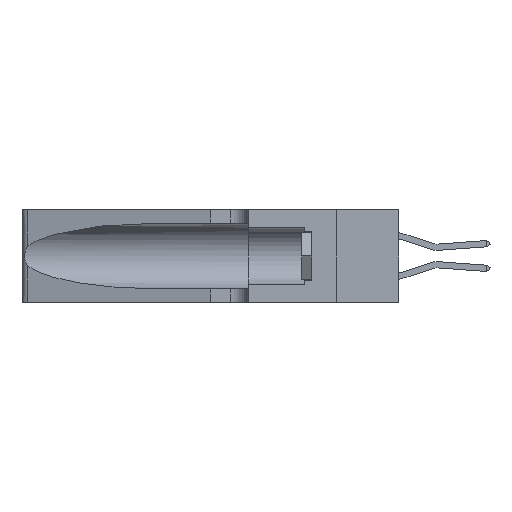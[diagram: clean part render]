
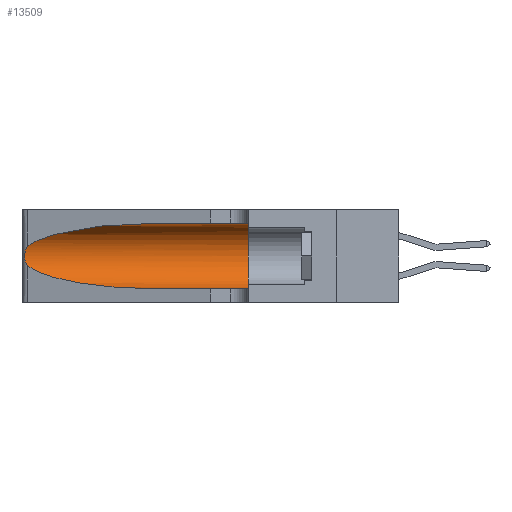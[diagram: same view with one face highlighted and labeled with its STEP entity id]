
A CAD part, left-side view. The second image highlights one B-rep face of the part: STEP entity #13509.
In plain terms, the highlighted cylindrical face has radius 3.308 mm (diameter 6.617 mm), a partial arc.
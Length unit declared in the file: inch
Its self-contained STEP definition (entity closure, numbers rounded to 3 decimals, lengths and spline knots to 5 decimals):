
#374 = DIRECTION ( 'NONE',  ( 0., 1., 0. ) ) ;
#683 = CARTESIAN_POINT ( 'NONE',  ( 0.1305, 1.61858, 0.185 ) ) ;
#778 = VERTEX_POINT ( 'NONE', #22351 ) ;
#1874 = CARTESIAN_POINT ( 'NONE',  ( 0.25555, 1.22994, 0.2215 ) ) ;
#3422 = ORIENTED_EDGE ( 'NONE', *, *, #38455, .T. ) ;
#3432 = CARTESIAN_POINT ( 'NONE',  ( 0.2373, 1.15595, 0.08982 ) ) ;
#3746 = VECTOR ( 'NONE', #6434, 39.37008 ) ;
#4234 = DIRECTION ( 'NONE',  ( 0., 0., 1. ) ) ;
#4545 = CARTESIAN_POINT ( 'NONE',  ( 0.25487, 1.22718, 0.14631 ) ) ;
#4566 = CIRCLE ( 'NONE', #34608, 0.13025 ) ;
#4576 = VERTEX_POINT ( 'NONE', #33039 ) ;
#4696 = EDGE_CURVE ( 'NONE', #21674, #39257, #19799, .T. ) ;
#5268 = CARTESIAN_POINT ( 'NONE',  ( 0.25787, 1.23484, 0.2124 ) ) ;
#6434 = DIRECTION ( 'NONE',  ( 0., -1., 0. ) ) ;
#6679 = LINE ( 'NONE', #36848, #17743 ) ;
#8816 = CARTESIAN_POINT ( 'NONE',  ( 0.26075, 1.23896, 0.178 ) ) ;
#10215 = CARTESIAN_POINT ( 'NONE',  ( 0.2373, 1.15595, 0.28018 ) ) ;
#10516 = CARTESIAN_POINT ( 'NONE',  ( 0.25487, 1.22718, 0.22369 ) ) ;
#10837 = CARTESIAN_POINT ( 'NONE',  ( 0.18966, 0.96281, 0.31525 ) ) ;
#10876 = EDGE_CURVE ( 'NONE', #4576, #778, #28569, .T. ) ;
#11073 = CARTESIAN_POINT ( 'NONE',  ( 0.1305, 0.72297, 0.31525 ) ) ;
#11968 = CARTESIAN_POINT ( 'NONE',  ( 0.18966, 0.96281, 0.05475 ) ) ;
#12072 = CARTESIAN_POINT ( 'NONE',  ( 0.25856, 1.23593, 0.16098 ) ) ;
#12936 = CARTESIAN_POINT ( 'NONE',  ( 0.25487, 1.22718, 0.22369 ) ) ;
#13333 = FACE_OUTER_BOUND ( 'NONE', #25990, .T. ) ;
#13509 = ADVANCED_FACE ( 'NONE', ( #13333 ), #38615, .F. ) ;
#15390 = CARTESIAN_POINT ( 'NONE',  ( 0.1305, 0.35, 0.05475 ) ) ;
#15497 = CARTESIAN_POINT ( 'NONE',  ( 0.25639, 1.23184, 0.21858 ) ) ;
#17743 = VECTOR ( 'NONE', #33472, 39.37008 ) ;
#19041 = CARTESIAN_POINT ( 'NONE',  ( 0.25487, 1.22718, 0.14631 ) ) ;
#19723 = VERTEX_POINT ( 'NONE', #20921 ) ;
#19799 =( BOUNDED_CURVE ( )  B_SPLINE_CURVE ( 3, ( #21370, #10837, #10215, #10516 ),
 .UNSPECIFIED., .F., .F. ) 
 B_SPLINE_CURVE_WITH_KNOTS ( ( 4, 4 ),
 ( 1.5708, 2.84003 ),
 .UNSPECIFIED. ) 
 CURVE ( )  GEOMETRIC_REPRESENTATION_ITEM ( )  RATIONAL_B_SPLINE_CURVE ( ( 1., 0.87, 0.87, 1. ) ) 
 REPRESENTATION_ITEM ( '' )  );
#20921 = CARTESIAN_POINT ( 'NONE',  ( 0.1305, 0.35, 0.31525 ) ) ;
#21370 = CARTESIAN_POINT ( 'NONE',  ( 0.1305, 0.72297, 0.31525 ) ) ;
#21674 = VERTEX_POINT ( 'NONE', #11073 ) ;
#22351 = CARTESIAN_POINT ( 'NONE',  ( 0.1305, 0.72297, 0.05475 ) ) ;
#25381 = DIRECTION ( 'NONE',  ( 0., 0., -1. ) ) ;
#25990 = EDGE_LOOP ( 'NONE', ( #37197, #3422, #37677, #34176, #37445, #29394 ) ) ;
#26283 = CARTESIAN_POINT ( 'NONE',  ( 0.26075, 1.23896, 0.19203 ) ) ;
#26728 = CARTESIAN_POINT ( 'NONE',  ( 0.26018, 1.23835, 0.19895 ) ) ;
#28569 =( BOUNDED_CURVE ( )  B_SPLINE_CURVE ( 3, ( #4545, #3432, #11968, #43664 ),
 .UNSPECIFIED., .F., .F. ) 
 B_SPLINE_CURVE_WITH_KNOTS ( ( 4, 4 ),
 ( 3.44316, 4.71239 ),
 .UNSPECIFIED. ) 
 CURVE ( )  GEOMETRIC_REPRESENTATION_ITEM ( )  RATIONAL_B_SPLINE_CURVE ( ( 1., 0.87, 0.87, 1. ) ) 
 REPRESENTATION_ITEM ( '' )  );
#29394 = ORIENTED_EDGE ( 'NONE', *, *, #44924, .F. ) ;
#29970 = EDGE_CURVE ( 'NONE', #778, #40865, #6679, .T. ) ;
#30265 = CARTESIAN_POINT ( 'NONE',  ( 0.25789, 1.23486, 0.15765 ) ) ;
#31355 = B_SPLINE_CURVE_WITH_KNOTS ( 'NONE', 3,
 ( #40667, #1874, #15497, #5268, #44218, #26728, #26283, #8816, #37175, #12072, #30265, #36582, #36875, #19041 ),
 .UNSPECIFIED., .F., .F.,
 ( 4, 2, 2, 2, 2, 2, 4 ),
 ( 0., 0.00027, 0.00053, 0.00107, 0.0016, 0.00187, 0.00214 ),
 .UNSPECIFIED. ) ;
#31583 = CARTESIAN_POINT ( 'NONE',  ( 0.1305, 1.61858, 0.31525 ) ) ;
#32644 = CARTESIAN_POINT ( 'NONE',  ( 0.1305, 0.35, 0.185 ) ) ;
#33039 = CARTESIAN_POINT ( 'NONE',  ( 0.25487, 1.22718, 0.14631 ) ) ;
#33065 = LINE ( 'NONE', #31583, #3746 ) ;
#33472 = DIRECTION ( 'NONE',  ( 0., -1., 0. ) ) ;
#33950 = AXIS2_PLACEMENT_3D ( 'NONE', #683, #43206, #25381 ) ;
#34176 = ORIENTED_EDGE ( 'NONE', *, *, #29970, .T. ) ;
#34608 = AXIS2_PLACEMENT_3D ( 'NONE', #32644, #374, #4234 ) ;
#36582 = CARTESIAN_POINT ( 'NONE',  ( 0.25639, 1.23186, 0.15144 ) ) ;
#36848 = CARTESIAN_POINT ( 'NONE',  ( 0.1305, 1.61858, 0.05475 ) ) ;
#36875 = CARTESIAN_POINT ( 'NONE',  ( 0.25555, 1.22993, 0.14849 ) ) ;
#37175 = CARTESIAN_POINT ( 'NONE',  ( 0.26017, 1.23833, 0.17102 ) ) ;
#37197 = ORIENTED_EDGE ( 'NONE', *, *, #4696, .T. ) ;
#37445 = ORIENTED_EDGE ( 'NONE', *, *, #42729, .F. ) ;
#37677 = ORIENTED_EDGE ( 'NONE', *, *, #10876, .T. ) ;
#38455 = EDGE_CURVE ( 'NONE', #39257, #4576, #31355, .T. ) ;
#38615 = CYLINDRICAL_SURFACE ( 'NONE', #33950, 0.13025 ) ;
#39257 = VERTEX_POINT ( 'NONE', #12936 ) ;
#40667 = CARTESIAN_POINT ( 'NONE',  ( 0.25487, 1.22718, 0.22369 ) ) ;
#40865 = VERTEX_POINT ( 'NONE', #15390 ) ;
#42729 = EDGE_CURVE ( 'NONE', #19723, #40865, #4566, .T. ) ;
#43206 = DIRECTION ( 'NONE',  ( 0., -1., 0. ) ) ;
#43664 = CARTESIAN_POINT ( 'NONE',  ( 0.1305, 0.72297, 0.05475 ) ) ;
#44218 = CARTESIAN_POINT ( 'NONE',  ( 0.25854, 1.2359, 0.20912 ) ) ;
#44924 = EDGE_CURVE ( 'NONE', #21674, #19723, #33065, .T. ) ;
